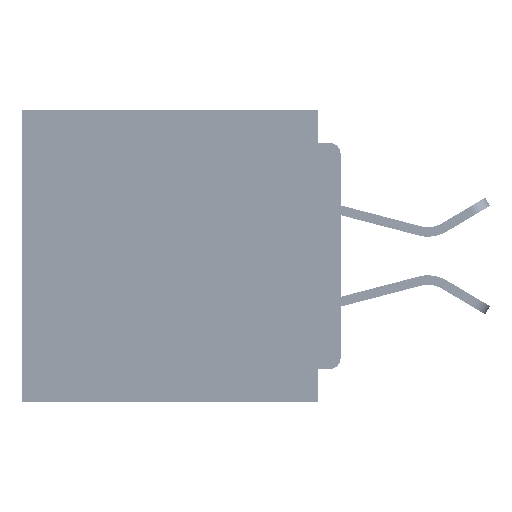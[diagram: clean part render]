
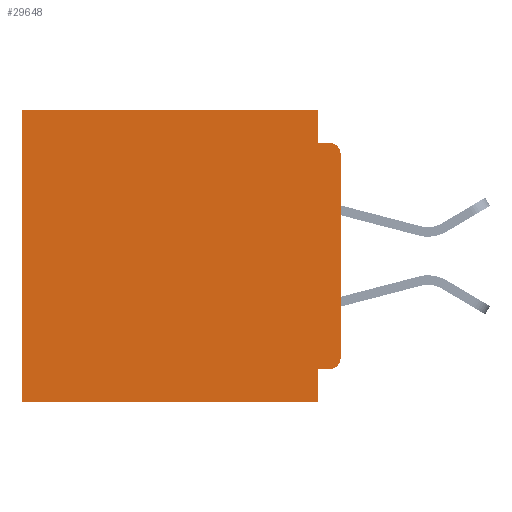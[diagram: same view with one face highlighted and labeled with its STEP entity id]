
A CAD part, left-side view. The second image highlights one B-rep face of the part: STEP entity #29648.
In plain terms, the highlighted planar face has unit normal (-1, 0, 0).
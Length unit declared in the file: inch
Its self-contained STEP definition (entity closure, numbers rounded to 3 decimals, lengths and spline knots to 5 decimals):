
#10 = DIRECTION ( 'NONE',  ( 0., -1., 0. ) ) ;
#35 = EDGE_CURVE ( 'NONE', #13383, #65098, #24192, .T. ) ;
#356 = AXIS2_PLACEMENT_3D ( 'NONE', #20528, #56204, #25658 ) ;
#647 = VERTEX_POINT ( 'NONE', #4600 ) ;
#1843 = VECTOR ( 'NONE', #36887, 39.37008 ) ;
#3647 = VERTEX_POINT ( 'NONE', #38205 ) ;
#4159 = VERTEX_POINT ( 'NONE', #27280 ) ;
#4600 = CARTESIAN_POINT ( 'NONE',  ( 0.3, 0.437, 0. ) ) ;
#5177 = EDGE_CURVE ( 'NONE', #65098, #4159, #57067, .T. ) ;
#6125 = CARTESIAN_POINT ( 'NONE',  ( 0.3, 0., -0.4 ) ) ;
#9495 = EDGE_CURVE ( 'NONE', #54063, #26718, #14643, .T. ) ;
#10615 = AXIS2_PLACEMENT_3D ( 'NONE', #46594, #16059, #51728 ) ;
#12206 = ORIENTED_EDGE ( 'NONE', *, *, #40084, .F. ) ;
#13097 = FACE_OUTER_BOUND ( 'NONE', #28758, .T. ) ;
#13206 = DIRECTION ( 'NONE',  ( 0., 1., 0. ) ) ;
#13383 = VERTEX_POINT ( 'NONE', #60698 ) ;
#14643 = LINE ( 'NONE', #6125, #28235 ) ;
#15078 = CARTESIAN_POINT ( 'NONE',  ( 0.3, 0.031, -0.4 ) ) ;
#16059 = DIRECTION ( 'NONE',  ( -1., 0., 0. ) ) ;
#17637 = EDGE_CURVE ( 'NONE', #3647, #32814, #65427, .T. ) ;
#19364 = ORIENTED_EDGE ( 'NONE', *, *, #44480, .T. ) ;
#20222 = DIRECTION ( 'NONE',  ( 0., 0., -1. ) ) ;
#20528 = CARTESIAN_POINT ( 'NONE',  ( 0.3, 0.015, -0.34 ) ) ;
#20751 = CARTESIAN_POINT ( 'NONE',  ( 0.3, 0.437, -0.4 ) ) ;
#22605 = VECTOR ( 'NONE', #57401, 39.37008 ) ;
#24192 = LINE ( 'NONE', #30984, #22605 ) ;
#25658 = DIRECTION ( 'NONE',  ( 0., 0., -1. ) ) ;
#25788 = VERTEX_POINT ( 'NONE', #27117 ) ;
#26656 = CARTESIAN_POINT ( 'NONE',  ( 0.3, 0., -0.4 ) ) ;
#26718 = VERTEX_POINT ( 'NONE', #49065 ) ;
#27117 = CARTESIAN_POINT ( 'NONE',  ( 0.3, 0.031, 0. ) ) ;
#27280 = CARTESIAN_POINT ( 'NONE',  ( 0.3, 0.031, -0.4 ) ) ;
#27862 = CIRCLE ( 'NONE', #356, 0.015 ) ;
#28095 = EDGE_CURVE ( 'NONE', #647, #55159, #43531, .T. ) ;
#28235 = VECTOR ( 'NONE', #41820, 39.37008 ) ;
#28691 = VECTOR ( 'NONE', #13206, 39.37008 ) ;
#28758 = EDGE_LOOP ( 'NONE', ( #31360, #19364, #32959, #12206, #39308, #32192, #38541, #52132, #55303, #56935 ) ) ;
#29648 = ADVANCED_FACE ( 'NONE', ( #13097 ), #50652, .F. ) ;
#30392 = DIRECTION ( 'NONE',  ( 0., 0., -1. ) ) ;
#30984 = CARTESIAN_POINT ( 'NONE',  ( 0.3, 0., -0.355 ) ) ;
#31360 = ORIENTED_EDGE ( 'NONE', *, *, #9495, .F. ) ;
#32192 = ORIENTED_EDGE ( 'NONE', *, *, #28095, .T. ) ;
#32515 = CARTESIAN_POINT ( 'NONE',  ( 0.3, 0., -0.06 ) ) ;
#32814 = VERTEX_POINT ( 'NONE', #51441 ) ;
#32959 = ORIENTED_EDGE ( 'NONE', *, *, #17637, .F. ) ;
#33494 = DIRECTION ( 'NONE',  ( 0., 0., -1. ) ) ;
#33521 = CARTESIAN_POINT ( 'NONE',  ( 0.3, 0., 0. ) ) ;
#36719 = VECTOR ( 'NONE', #10, 39.37008 ) ;
#36887 = DIRECTION ( 'NONE',  ( 0., 1., 0. ) ) ;
#38205 = CARTESIAN_POINT ( 'NONE',  ( 0.3, 0.031, -0.045 ) ) ;
#38541 = ORIENTED_EDGE ( 'NONE', *, *, #39143, .F. ) ;
#39143 = EDGE_CURVE ( 'NONE', #4159, #55159, #40948, .T. ) ;
#39308 = ORIENTED_EDGE ( 'NONE', *, *, #44094, .T. ) ;
#40084 = EDGE_CURVE ( 'NONE', #25788, #3647, #40814, .T. ) ;
#40814 = LINE ( 'NONE', #50366, #63173 ) ;
#40948 = LINE ( 'NONE', #26656, #1843 ) ;
#41820 = DIRECTION ( 'NONE',  ( 0., 0., -1. ) ) ;
#42246 = LINE ( 'NONE', #33521, #28691 ) ;
#43484 = VECTOR ( 'NONE', #20222, 39.37008 ) ;
#43531 = LINE ( 'NONE', #58897, #58715 ) ;
#44094 = EDGE_CURVE ( 'NONE', #25788, #647, #42246, .T. ) ;
#44379 = EDGE_CURVE ( 'NONE', #13383, #26718, #27862, .T. ) ;
#44480 = EDGE_CURVE ( 'NONE', #54063, #32814, #60546, .T. ) ;
#45523 = CARTESIAN_POINT ( 'NONE',  ( 0.3, 0., -0.4 ) ) ;
#46224 = AXIS2_PLACEMENT_3D ( 'NONE', #45523, #60924, #30392 ) ;
#46594 = CARTESIAN_POINT ( 'NONE',  ( 0.3, 0.015, -0.06 ) ) ;
#49065 = CARTESIAN_POINT ( 'NONE',  ( 0.3, 0., -0.34 ) ) ;
#50366 = CARTESIAN_POINT ( 'NONE',  ( 0.3, 0.031, 0. ) ) ;
#50652 = PLANE ( 'NONE',  #46224 ) ;
#51441 = CARTESIAN_POINT ( 'NONE',  ( 0.3, 0.015, -0.045 ) ) ;
#51728 = DIRECTION ( 'NONE',  ( 0., 0., -1. ) ) ;
#52132 = ORIENTED_EDGE ( 'NONE', *, *, #5177, .F. ) ;
#53486 = CARTESIAN_POINT ( 'NONE',  ( 0.3, 0.031, -0.355 ) ) ;
#54063 = VERTEX_POINT ( 'NONE', #32515 ) ;
#55159 = VERTEX_POINT ( 'NONE', #20751 ) ;
#55303 = ORIENTED_EDGE ( 'NONE', *, *, #35, .F. ) ;
#55515 = DIRECTION ( 'NONE',  ( 0., 0., -1. ) ) ;
#56204 = DIRECTION ( 'NONE',  ( -1., 0., 0. ) ) ;
#56935 = ORIENTED_EDGE ( 'NONE', *, *, #44379, .T. ) ;
#57067 = LINE ( 'NONE', #15078, #43484 ) ;
#57401 = DIRECTION ( 'NONE',  ( 0., 1., 0. ) ) ;
#58715 = VECTOR ( 'NONE', #33494, 39.37008 ) ;
#58897 = CARTESIAN_POINT ( 'NONE',  ( 0.3, 0.437, -0.4 ) ) ;
#60546 = CIRCLE ( 'NONE', #10615, 0.015 ) ;
#60698 = CARTESIAN_POINT ( 'NONE',  ( 0.3, 0.015, -0.355 ) ) ;
#60924 = DIRECTION ( 'NONE',  ( 1., 0., 0. ) ) ;
#63173 = VECTOR ( 'NONE', #55515, 39.37008 ) ;
#65098 = VERTEX_POINT ( 'NONE', #53486 ) ;
#65427 = LINE ( 'NONE', #66017, #36719 ) ;
#66017 = CARTESIAN_POINT ( 'NONE',  ( 0.3, 0., -0.045 ) ) ;
